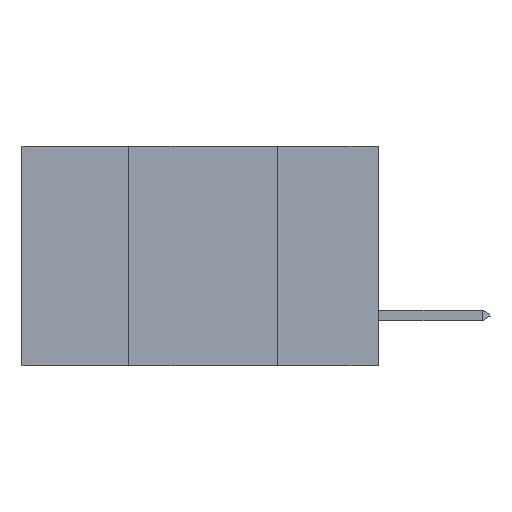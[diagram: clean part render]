
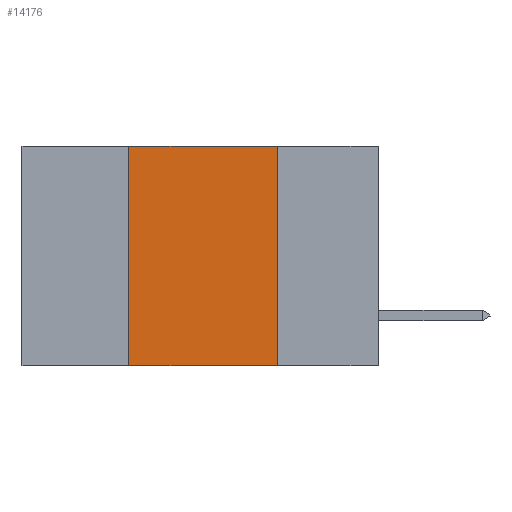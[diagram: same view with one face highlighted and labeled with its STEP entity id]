
A CAD part, left-side view. The second image highlights one B-rep face of the part: STEP entity #14176.
In plain terms, the highlighted planar face has unit normal (-1, 0, 0).
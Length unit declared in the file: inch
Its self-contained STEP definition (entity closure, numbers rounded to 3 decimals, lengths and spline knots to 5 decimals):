
#79 = VECTOR ( 'NONE', #366, 39.37008 ) ;
#182 = CARTESIAN_POINT ( 'NONE',  ( 0., 0.17, 0. ) ) ;
#366 = DIRECTION ( 'NONE',  ( 0., 0., -1. ) ) ;
#582 = VECTOR ( 'NONE', #13082, 39.37008 ) ;
#1524 = EDGE_CURVE ( 'NONE', #3864, #10927, #15795, .T. ) ;
#2620 = LINE ( 'NONE', #11148, #3866 ) ;
#3659 = LINE ( 'NONE', #10119, #19885 ) ;
#3687 = CARTESIAN_POINT ( 'NONE',  ( 0., 0.17, 0. ) ) ;
#3831 = FACE_OUTER_BOUND ( 'NONE', #16818, .T. ) ;
#3864 = VERTEX_POINT ( 'NONE', #20112 ) ;
#3866 = VECTOR ( 'NONE', #8093, 39.37008 ) ;
#3868 = DIRECTION ( 'NONE',  ( 0., -1., 0. ) ) ;
#4847 = EDGE_CURVE ( 'NONE', #9231, #7380, #3659, .T. ) ;
#6970 = ORIENTED_EDGE ( 'NONE', *, *, #1524, .F. ) ;
#7380 = VERTEX_POINT ( 'NONE', #18659 ) ;
#8093 = DIRECTION ( 'NONE',  ( 0., 0., 1. ) ) ;
#8346 = CARTESIAN_POINT ( 'NONE',  ( 0., 0.42, -0.37 ) ) ;
#8497 = DIRECTION ( 'NONE',  ( 1., 0., 0. ) ) ;
#9231 = VERTEX_POINT ( 'NONE', #8346 ) ;
#9942 = LINE ( 'NONE', #3687, #79 ) ;
#10119 = CARTESIAN_POINT ( 'NONE',  ( 0., 0.6, -0.37 ) ) ;
#10927 = VERTEX_POINT ( 'NONE', #182 ) ;
#11148 = CARTESIAN_POINT ( 'NONE',  ( 0., 0.42, 0. ) ) ;
#11534 = DIRECTION ( 'NONE',  ( 0., 0., -1. ) ) ;
#11673 = CARTESIAN_POINT ( 'NONE',  ( 0., 0.6, 0. ) ) ;
#12499 = ORIENTED_EDGE ( 'NONE', *, *, #14689, .F. ) ;
#13082 = DIRECTION ( 'NONE',  ( 0., -1., 0. ) ) ;
#13257 = EDGE_CURVE ( 'NONE', #9231, #3864, #2620, .T. ) ;
#14176 = ADVANCED_FACE ( 'NONE', ( #3831 ), #14815, .F. ) ;
#14689 = EDGE_CURVE ( 'NONE', #10927, #7380, #9942, .T. ) ;
#14815 = PLANE ( 'NONE',  #18232 ) ;
#15795 = LINE ( 'NONE', #17714, #582 ) ;
#16310 = ORIENTED_EDGE ( 'NONE', *, *, #4847, .T. ) ;
#16818 = EDGE_LOOP ( 'NONE', ( #12499, #6970, #19734, #16310 ) ) ;
#17714 = CARTESIAN_POINT ( 'NONE',  ( 0., 0.6, 0. ) ) ;
#18232 = AXIS2_PLACEMENT_3D ( 'NONE', #11673, #8497, #11534 ) ;
#18659 = CARTESIAN_POINT ( 'NONE',  ( 0., 0.17, -0.37 ) ) ;
#19734 = ORIENTED_EDGE ( 'NONE', *, *, #13257, .F. ) ;
#19885 = VECTOR ( 'NONE', #3868, 39.37008 ) ;
#20112 = CARTESIAN_POINT ( 'NONE',  ( 0., 0.42, 0. ) ) ;
